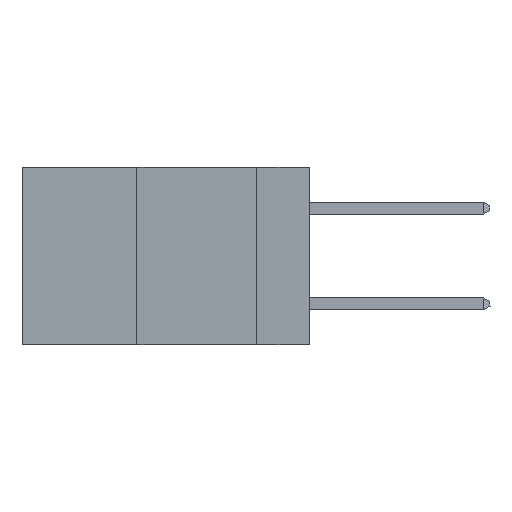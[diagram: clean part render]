
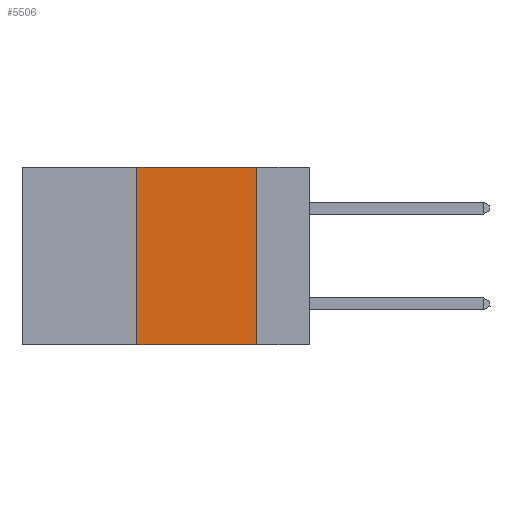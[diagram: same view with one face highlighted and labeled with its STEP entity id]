
A CAD part, left-side view. The second image highlights one B-rep face of the part: STEP entity #5506.
In plain terms, the highlighted planar face has unit normal (-1, 0, 0).
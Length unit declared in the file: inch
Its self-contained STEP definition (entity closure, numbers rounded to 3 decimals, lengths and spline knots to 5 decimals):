
#584 = VERTEX_POINT ( 'NONE', #11490 ) ;
#1298 = CARTESIAN_POINT ( 'NONE',  ( 0., 0.6, 0. ) ) ;
#1571 = EDGE_CURVE ( 'NONE', #584, #8605, #10092, .T. ) ;
#1735 = DIRECTION ( 'NONE',  ( 0., -1., 0. ) ) ;
#1877 = VERTEX_POINT ( 'NONE', #9757 ) ;
#2999 = DIRECTION ( 'NONE',  ( 0., 0., -1. ) ) ;
#3024 = CARTESIAN_POINT ( 'NONE',  ( 0., 0.11, 0. ) ) ;
#4716 = VECTOR ( 'NONE', #1735, 39.37008 ) ;
#4862 = CARTESIAN_POINT ( 'NONE',  ( 0., 0.36, -0.37 ) ) ;
#5506 = ADVANCED_FACE ( 'NONE', ( #11319 ), #7532, .F. ) ;
#5677 = AXIS2_PLACEMENT_3D ( 'NONE', #17646, #9198, #20967 ) ;
#6348 = VERTEX_POINT ( 'NONE', #4862 ) ;
#6475 = VECTOR ( 'NONE', #20907, 39.37008 ) ;
#7532 = PLANE ( 'NONE',  #5677 ) ;
#8208 = EDGE_LOOP ( 'NONE', ( #13084, #13852, #14624, #15057 ) ) ;
#8605 = VERTEX_POINT ( 'NONE', #10760 ) ;
#9120 = LINE ( 'NONE', #18658, #4716 ) ;
#9198 = DIRECTION ( 'NONE',  ( 1., 0., 0. ) ) ;
#9757 = CARTESIAN_POINT ( 'NONE',  ( 0., 0.36, 0. ) ) ;
#9858 = EDGE_CURVE ( 'NONE', #6348, #1877, #10837, .T. ) ;
#10092 = LINE ( 'NONE', #3024, #18585 ) ;
#10760 = CARTESIAN_POINT ( 'NONE',  ( 0., 0.11, -0.37 ) ) ;
#10837 = LINE ( 'NONE', #15829, #6475 ) ;
#11319 = FACE_OUTER_BOUND ( 'NONE', #8208, .T. ) ;
#11490 = CARTESIAN_POINT ( 'NONE',  ( 0., 0.11, 0. ) ) ;
#13084 = ORIENTED_EDGE ( 'NONE', *, *, #1571, .F. ) ;
#13193 = DIRECTION ( 'NONE',  ( 0., -1., 0. ) ) ;
#13852 = ORIENTED_EDGE ( 'NONE', *, *, #18933, .F. ) ;
#14624 = ORIENTED_EDGE ( 'NONE', *, *, #9858, .F. ) ;
#15057 = ORIENTED_EDGE ( 'NONE', *, *, #19760, .T. ) ;
#15829 = CARTESIAN_POINT ( 'NONE',  ( 0., 0.36, 0. ) ) ;
#17646 = CARTESIAN_POINT ( 'NONE',  ( 0., 0.6, 0. ) ) ;
#17647 = LINE ( 'NONE', #1298, #21520 ) ;
#18585 = VECTOR ( 'NONE', #2999, 39.37008 ) ;
#18658 = CARTESIAN_POINT ( 'NONE',  ( 0., 0.6, -0.37 ) ) ;
#18933 = EDGE_CURVE ( 'NONE', #1877, #584, #17647, .T. ) ;
#19760 = EDGE_CURVE ( 'NONE', #6348, #8605, #9120, .T. ) ;
#20907 = DIRECTION ( 'NONE',  ( 0., 0., 1. ) ) ;
#20967 = DIRECTION ( 'NONE',  ( 0., 0., -1. ) ) ;
#21520 = VECTOR ( 'NONE', #13193, 39.37008 ) ;
